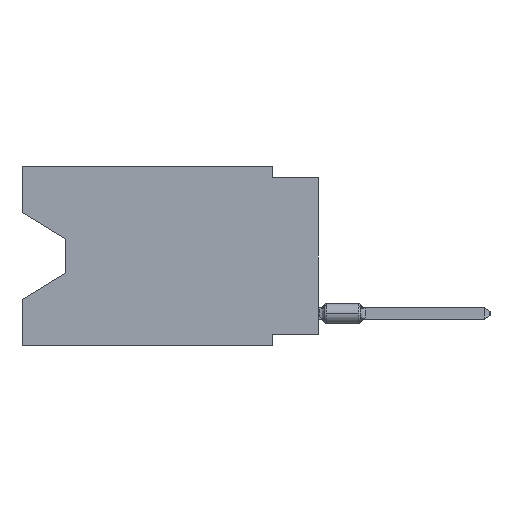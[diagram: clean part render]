
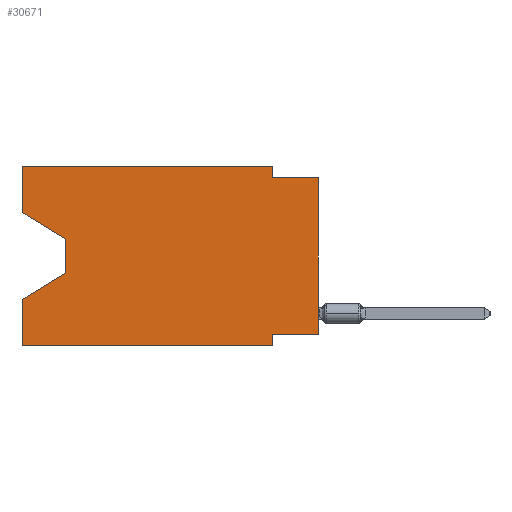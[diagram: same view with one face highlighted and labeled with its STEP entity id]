
A CAD part, left-side view. The second image highlights one B-rep face of the part: STEP entity #30671.
In plain terms, the highlighted planar face has unit normal (-1, 0, 0).
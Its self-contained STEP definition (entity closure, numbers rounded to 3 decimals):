
#781 = ORIENTED_EDGE ( 'NONE', *, *, #40133, .T. ) ;
#1113 = ORIENTED_EDGE ( 'NONE', *, *, #12674, .F. ) ;
#2264 = ORIENTED_EDGE ( 'NONE', *, *, #41177, .F. ) ;
#3076 = VERTEX_POINT ( 'NONE', #38572 ) ;
#3143 = ORIENTED_EDGE ( 'NONE', *, *, #47341, .F. ) ;
#3175 = CARTESIAN_POINT ( 'NONE',  ( 0., 13.97, -4.013 ) ) ;
#3378 = DIRECTION ( 'NONE',  ( 0., 0.855, -0.519 ) ) ;
#3622 = VECTOR ( 'NONE', #4666, 1000. ) ;
#4122 = CARTESIAN_POINT ( 'NONE',  ( 0., 13.97, -5.893 ) ) ;
#4407 = CARTESIAN_POINT ( 'NONE',  ( 0., 2.54, 0. ) ) ;
#4423 = LINE ( 'NONE', #45549, #3622 ) ;
#4666 = DIRECTION ( 'NONE',  ( 0., 1., 0. ) ) ;
#5158 = VECTOR ( 'NONE', #10110, 1000. ) ;
#5392 = DIRECTION ( 'NONE',  ( 0., 0., -1. ) ) ;
#6141 = VERTEX_POINT ( 'NONE', #24227 ) ;
#6357 = CARTESIAN_POINT ( 'NONE',  ( 0., 2.54, -0.635 ) ) ;
#7036 = CARTESIAN_POINT ( 'NONE',  ( 0., 13.97, -5.893 ) ) ;
#7043 = EDGE_CURVE ( 'NONE', #44816, #21942, #14563, .T. ) ;
#7331 = CARTESIAN_POINT ( 'NONE',  ( 0., 16.383, -9.906 ) ) ;
#7439 = VERTEX_POINT ( 'NONE', #7331 ) ;
#7738 = LINE ( 'NONE', #29762, #43664 ) ;
#8084 = ORIENTED_EDGE ( 'NONE', *, *, #32242, .T. ) ;
#8757 = CARTESIAN_POINT ( 'NONE',  ( 0., 16.383, -7.36 ) ) ;
#8791 = EDGE_CURVE ( 'NONE', #13283, #26677, #33503, .T. ) ;
#10110 = DIRECTION ( 'NONE',  ( 0., 0., 1. ) ) ;
#10782 = EDGE_CURVE ( 'NONE', #15459, #43760, #29269, .T. ) ;
#10888 = CARTESIAN_POINT ( 'NONE',  ( 0., 0., -0.635 ) ) ;
#12242 = VERTEX_POINT ( 'NONE', #8757 ) ;
#12627 = CARTESIAN_POINT ( 'NONE',  ( 0., 2.54, -9.906 ) ) ;
#12674 = EDGE_CURVE ( 'NONE', #6141, #39231, #4423, .T. ) ;
#12957 = EDGE_CURVE ( 'NONE', #7439, #12242, #36205, .T. ) ;
#13060 = VECTOR ( 'NONE', #39783, 1000. ) ;
#13283 = VERTEX_POINT ( 'NONE', #42539 ) ;
#14321 = LINE ( 'NONE', #21172, #33054 ) ;
#14401 = EDGE_CURVE ( 'NONE', #24033, #13283, #16836, .T. ) ;
#14563 = LINE ( 'NONE', #10888, #13060 ) ;
#14700 = EDGE_CURVE ( 'NONE', #6141, #21942, #7738, .T. ) ;
#15084 = CARTESIAN_POINT ( 'NONE',  ( 0., 16.383, 0. ) ) ;
#15459 = VERTEX_POINT ( 'NONE', #18161 ) ;
#16836 = LINE ( 'NONE', #27823, #35785 ) ;
#18161 = CARTESIAN_POINT ( 'NONE',  ( 0., 16.383, 0. ) ) ;
#19329 = DIRECTION ( 'NONE',  ( 0., 0., -1. ) ) ;
#19361 = DIRECTION ( 'NONE',  ( 1., 0., 0. ) ) ;
#20713 = AXIS2_PLACEMENT_3D ( 'NONE', #35008, #19361, #5392 ) ;
#20936 = DIRECTION ( 'NONE',  ( 0., 0., -1. ) ) ;
#21172 = CARTESIAN_POINT ( 'NONE',  ( 0., 16.383, -9.906 ) ) ;
#21942 = VERTEX_POINT ( 'NONE', #44431 ) ;
#22122 = EDGE_LOOP ( 'NONE', ( #42372, #34154, #8084, #48302, #781, #2264, #1113, #29784, #41820, #3143, #28385, #37053 ) ) ;
#22169 = DIRECTION ( 'NONE',  ( 0., -1., 0. ) ) ;
#22199 = VECTOR ( 'NONE', #22169, 1000. ) ;
#22667 = DIRECTION ( 'NONE',  ( 0., 0., 1. ) ) ;
#23919 = DIRECTION ( 'NONE',  ( 0., -0.855, -0.519 ) ) ;
#24033 = VERTEX_POINT ( 'NONE', #39676 ) ;
#24227 = CARTESIAN_POINT ( 'NONE',  ( 0., 0., -9.271 ) ) ;
#24935 = VECTOR ( 'NONE', #40368, 1000. ) ;
#26677 = VERTEX_POINT ( 'NONE', #4122 ) ;
#27823 = CARTESIAN_POINT ( 'NONE',  ( 0., 16.383, -2.546 ) ) ;
#28385 = ORIENTED_EDGE ( 'NONE', *, *, #10782, .F. ) ;
#29269 = LINE ( 'NONE', #15084, #22199 ) ;
#29709 = DIRECTION ( 'NONE',  ( 0., -1., 0. ) ) ;
#29762 = CARTESIAN_POINT ( 'NONE',  ( 0., 0., 0. ) ) ;
#29784 = ORIENTED_EDGE ( 'NONE', *, *, #14700, .T. ) ;
#30671 = ADVANCED_FACE ( 'NONE', ( #41880 ), #34532, .F. ) ;
#32191 = CARTESIAN_POINT ( 'NONE',  ( 0., 2.54, 0. ) ) ;
#32242 = EDGE_CURVE ( 'NONE', #26677, #12242, #44251, .T. ) ;
#32373 = VECTOR ( 'NONE', #3378, 1000. ) ;
#33054 = VECTOR ( 'NONE', #29709, 1000. ) ;
#33503 = LINE ( 'NONE', #3175, #24935 ) ;
#34154 = ORIENTED_EDGE ( 'NONE', *, *, #8791, .T. ) ;
#34220 = EDGE_CURVE ( 'NONE', #24033, #15459, #40464, .T. ) ;
#34532 = PLANE ( 'NONE',  #20713 ) ;
#35008 = CARTESIAN_POINT ( 'NONE',  ( 0., 16.383, 0. ) ) ;
#35785 = VECTOR ( 'NONE', #23919, 1000. ) ;
#35962 = CARTESIAN_POINT ( 'NONE',  ( 0., 16.383, 0. ) ) ;
#36205 = LINE ( 'NONE', #35962, #37266 ) ;
#36210 = CARTESIAN_POINT ( 'NONE',  ( 0., 2.54, -9.271 ) ) ;
#36689 = DIRECTION ( 'NONE',  ( 0., 0., 1. ) ) ;
#37053 = ORIENTED_EDGE ( 'NONE', *, *, #34220, .F. ) ;
#37266 = VECTOR ( 'NONE', #36689, 1000. ) ;
#37934 = LINE ( 'NONE', #4407, #43882 ) ;
#38572 = CARTESIAN_POINT ( 'NONE',  ( 0., 2.54, -9.906 ) ) ;
#38818 = LINE ( 'NONE', #12627, #45536 ) ;
#39231 = VERTEX_POINT ( 'NONE', #36210 ) ;
#39676 = CARTESIAN_POINT ( 'NONE',  ( 0., 16.383, -2.546 ) ) ;
#39783 = DIRECTION ( 'NONE',  ( 0., -1., 0. ) ) ;
#40133 = EDGE_CURVE ( 'NONE', #7439, #3076, #14321, .T. ) ;
#40368 = DIRECTION ( 'NONE',  ( 0., 0., -1. ) ) ;
#40464 = LINE ( 'NONE', #43177, #5158 ) ;
#41177 = EDGE_CURVE ( 'NONE', #39231, #3076, #38818, .T. ) ;
#41820 = ORIENTED_EDGE ( 'NONE', *, *, #7043, .F. ) ;
#41880 = FACE_OUTER_BOUND ( 'NONE', #22122, .T. ) ;
#42372 = ORIENTED_EDGE ( 'NONE', *, *, #14401, .T. ) ;
#42539 = CARTESIAN_POINT ( 'NONE',  ( 0., 13.97, -4.013 ) ) ;
#43177 = CARTESIAN_POINT ( 'NONE',  ( 0., 16.383, 0. ) ) ;
#43664 = VECTOR ( 'NONE', #22667, 1000. ) ;
#43760 = VERTEX_POINT ( 'NONE', #32191 ) ;
#43882 = VECTOR ( 'NONE', #19329, 1000. ) ;
#44251 = LINE ( 'NONE', #7036, #32373 ) ;
#44431 = CARTESIAN_POINT ( 'NONE',  ( 0., 0., -0.635 ) ) ;
#44816 = VERTEX_POINT ( 'NONE', #6357 ) ;
#45536 = VECTOR ( 'NONE', #20936, 1000. ) ;
#45549 = CARTESIAN_POINT ( 'NONE',  ( 0., 0., -9.271 ) ) ;
#47341 = EDGE_CURVE ( 'NONE', #43760, #44816, #37934, .T. ) ;
#48302 = ORIENTED_EDGE ( 'NONE', *, *, #12957, .F. ) ;
